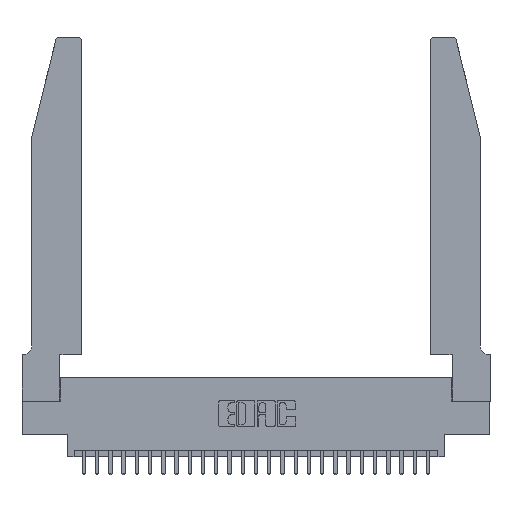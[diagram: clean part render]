
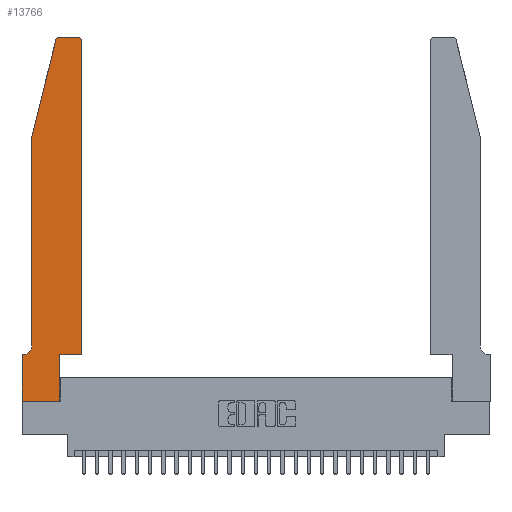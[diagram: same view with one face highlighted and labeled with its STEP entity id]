
A CAD part, top view. The second image highlights one B-rep face of the part: STEP entity #13766.
In plain terms, the highlighted planar face has unit normal (0, 0, 1).
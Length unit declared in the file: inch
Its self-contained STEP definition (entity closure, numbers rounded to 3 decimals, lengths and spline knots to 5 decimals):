
#180 = VECTOR ( 'NONE', #20791, 39.37008 ) ;
#349 = CARTESIAN_POINT ( 'NONE',  ( 0.0055, 0.35, 0.37 ) ) ;
#538 = DIRECTION ( 'NONE',  ( 0., 0., 1. ) ) ;
#613 = DIRECTION ( 'NONE',  ( -0.239, -0.971, 0. ) ) ;
#856 = CARTESIAN_POINT ( 'NONE',  ( 0.2605, 2.75, 0.37 ) ) ;
#1047 = EDGE_CURVE ( 'NONE', #24297, #16888, #28134, .T. ) ;
#1072 = DIRECTION ( 'NONE',  ( 0., 1., 0. ) ) ;
#1784 = CARTESIAN_POINT ( 'NONE',  ( 0., 0., 0.37 ) ) ;
#1854 = VECTOR ( 'NONE', #25260, 39.37008 ) ;
#2248 = EDGE_CURVE ( 'NONE', #17133, #15764, #22251, .T. ) ;
#2498 = VERTEX_POINT ( 'NONE', #10801 ) ;
#3468 = CIRCLE ( 'NONE', #11384, 0.03 ) ;
#3705 = DIRECTION ( 'NONE',  ( 1., 0., 0. ) ) ;
#4107 = AXIS2_PLACEMENT_3D ( 'NONE', #14179, #20721, #8037 ) ;
#4218 = CARTESIAN_POINT ( 'NONE',  ( 0.0755, 2., 0.37 ) ) ;
#4398 = EDGE_CURVE ( 'NONE', #16888, #2498, #3468, .T. ) ;
#4449 = CARTESIAN_POINT ( 'NONE',  ( 0.0755, 0.35, 0.37 ) ) ;
#4820 = VECTOR ( 'NONE', #8556, 39.37008 ) ;
#5289 = ORIENTED_EDGE ( 'NONE', *, *, #16369, .T. ) ;
#6304 = LINE ( 'NONE', #22009, #22930 ) ;
#6867 = CARTESIAN_POINT ( 'NONE',  ( 0., 0.35, 0.37 ) ) ;
#7314 = VECTOR ( 'NONE', #1072, 39.37008 ) ;
#7730 = CARTESIAN_POINT ( 'NONE',  ( 0.0755, 2., 0.37 ) ) ;
#8037 = DIRECTION ( 'NONE',  ( -1., 0., 0. ) ) ;
#8048 = VECTOR ( 'NONE', #26837, 39.37008 ) ;
#8246 = CARTESIAN_POINT ( 'NONE',  ( 0., 0.35, 0.37 ) ) ;
#8325 = VERTEX_POINT ( 'NONE', #9716 ) ;
#8399 = LINE ( 'NONE', #27541, #14498 ) ;
#8482 = DIRECTION ( 'NONE',  ( 1., 0., 0. ) ) ;
#8556 = DIRECTION ( 'NONE',  ( 1., 0., 0. ) ) ;
#8605 = ORIENTED_EDGE ( 'NONE', *, *, #16650, .T. ) ;
#9026 = CARTESIAN_POINT ( 'NONE',  ( 0.2865, 0.35, 0.37 ) ) ;
#9716 = CARTESIAN_POINT ( 'NONE',  ( 0.0755, 2., 0.37 ) ) ;
#9891 = CARTESIAN_POINT ( 'NONE',  ( 0.2865, 0., 0.37 ) ) ;
#10293 = ORIENTED_EDGE ( 'NONE', *, *, #2248, .T. ) ;
#10742 = LINE ( 'NONE', #20646, #8048 ) ;
#10801 = CARTESIAN_POINT ( 'NONE',  ( 0.25487, 2.72718, 0.37 ) ) ;
#10845 = ORIENTED_EDGE ( 'NONE', *, *, #22324, .T. ) ;
#10915 = ORIENTED_EDGE ( 'NONE', *, *, #21573, .T. ) ;
#11346 = CARTESIAN_POINT ( 'NONE',  ( 0.4205, 2.72, 0.37 ) ) ;
#11384 = AXIS2_PLACEMENT_3D ( 'NONE', #19476, #27945, #8482 ) ;
#11965 = EDGE_CURVE ( 'NONE', #21100, #16824, #18745, .T. ) ;
#12116 = ORIENTED_EDGE ( 'NONE', *, *, #24431, .T. ) ;
#12327 = VERTEX_POINT ( 'NONE', #9891 ) ;
#12569 = CARTESIAN_POINT ( 'NONE',  ( 0.284, 2.75, 0.37 ) ) ;
#13395 = LINE ( 'NONE', #4449, #1854 ) ;
#13766 = ADVANCED_FACE ( 'NONE', ( #23053 ), #27431, .T. ) ;
#14179 = CARTESIAN_POINT ( 'NONE',  ( 0.0055, 0.42, 0.37 ) ) ;
#14498 = VECTOR ( 'NONE', #27365, 39.37008 ) ;
#15276 = EDGE_CURVE ( 'NONE', #12327, #16425, #8399, .T. ) ;
#15707 = CIRCLE ( 'NONE', #15959, 0.03 ) ;
#15764 = VERTEX_POINT ( 'NONE', #24985 ) ;
#15841 = VECTOR ( 'NONE', #613, 39.37008 ) ;
#15959 = AXIS2_PLACEMENT_3D ( 'NONE', #11346, #538, #17813 ) ;
#16176 = VERTEX_POINT ( 'NONE', #6867 ) ;
#16369 = EDGE_CURVE ( 'NONE', #16176, #26821, #6304, .T. ) ;
#16425 = VERTEX_POINT ( 'NONE', #9026 ) ;
#16543 = ORIENTED_EDGE ( 'NONE', *, *, #1047, .T. ) ;
#16650 = EDGE_CURVE ( 'NONE', #16824, #16176, #13395, .T. ) ;
#16824 = VERTEX_POINT ( 'NONE', #349 ) ;
#16888 = VERTEX_POINT ( 'NONE', #12569 ) ;
#17133 = VERTEX_POINT ( 'NONE', #24877 ) ;
#17414 = ORIENTED_EDGE ( 'NONE', *, *, #11965, .T. ) ;
#17813 = DIRECTION ( 'NONE',  ( 1., 0., 0. ) ) ;
#18031 = LINE ( 'NONE', #23453, #4820 ) ;
#18745 = CIRCLE ( 'NONE', #4107, 0.07 ) ;
#19476 = CARTESIAN_POINT ( 'NONE',  ( 0.284, 2.72, 0.37 ) ) ;
#19830 = DIRECTION ( 'NONE',  ( 0., -1., 0. ) ) ;
#20646 = CARTESIAN_POINT ( 'NONE',  ( 0.4505, 0.35, 0.37 ) ) ;
#20721 = DIRECTION ( 'NONE',  ( 0., 0., -1. ) ) ;
#20791 = DIRECTION ( 'NONE',  ( 0., -1., 0. ) ) ;
#20929 = LINE ( 'NONE', #4218, #15841 ) ;
#20981 = VECTOR ( 'NONE', #26876, 39.37008 ) ;
#21100 = VERTEX_POINT ( 'NONE', #27762 ) ;
#21184 = CARTESIAN_POINT ( 'NONE',  ( 0.4205, 2.75, 0.37 ) ) ;
#21460 = EDGE_CURVE ( 'NONE', #2498, #8325, #20929, .T. ) ;
#21573 = EDGE_CURVE ( 'NONE', #16425, #17133, #10742, .T. ) ;
#22009 = CARTESIAN_POINT ( 'NONE',  ( 0., 0., 0.37 ) ) ;
#22251 = LINE ( 'NONE', #27095, #7314 ) ;
#22324 = EDGE_CURVE ( 'NONE', #8325, #21100, #28021, .T. ) ;
#22930 = VECTOR ( 'NONE', #19830, 39.37008 ) ;
#23053 = FACE_OUTER_BOUND ( 'NONE', #25169, .T. ) ;
#23130 = DIRECTION ( 'NONE',  ( 0., 0., 1. ) ) ;
#23453 = CARTESIAN_POINT ( 'NONE',  ( 0., 0., 0.37 ) ) ;
#24297 = VERTEX_POINT ( 'NONE', #21184 ) ;
#24431 = EDGE_CURVE ( 'NONE', #26821, #12327, #18031, .T. ) ;
#24877 = CARTESIAN_POINT ( 'NONE',  ( 0.4505, 0.35, 0.37 ) ) ;
#24985 = CARTESIAN_POINT ( 'NONE',  ( 0.4505, 2.72, 0.37 ) ) ;
#25169 = EDGE_LOOP ( 'NONE', ( #16543, #25795, #25271, #10845, #17414, #8605, #5289, #12116, #27319, #10915, #10293, #25614 ) ) ;
#25260 = DIRECTION ( 'NONE',  ( -1., 0., 0. ) ) ;
#25271 = ORIENTED_EDGE ( 'NONE', *, *, #21460, .T. ) ;
#25503 = EDGE_CURVE ( 'NONE', #15764, #24297, #15707, .T. ) ;
#25614 = ORIENTED_EDGE ( 'NONE', *, *, #25503, .T. ) ;
#25795 = ORIENTED_EDGE ( 'NONE', *, *, #4398, .T. ) ;
#26284 = AXIS2_PLACEMENT_3D ( 'NONE', #8246, #23130, #3705 ) ;
#26821 = VERTEX_POINT ( 'NONE', #1784 ) ;
#26837 = DIRECTION ( 'NONE',  ( 1., 0., 0. ) ) ;
#26876 = DIRECTION ( 'NONE',  ( -1., 0., 0. ) ) ;
#27095 = CARTESIAN_POINT ( 'NONE',  ( 0.4505, 0.35, 0.37 ) ) ;
#27319 = ORIENTED_EDGE ( 'NONE', *, *, #15276, .T. ) ;
#27365 = DIRECTION ( 'NONE',  ( 0., 1., 0. ) ) ;
#27431 = PLANE ( 'NONE',  #26284 ) ;
#27541 = CARTESIAN_POINT ( 'NONE',  ( 0.2865, 0.35, 0.37 ) ) ;
#27762 = CARTESIAN_POINT ( 'NONE',  ( 0.0755, 0.42, 0.37 ) ) ;
#27945 = DIRECTION ( 'NONE',  ( 0., 0., 1. ) ) ;
#28021 = LINE ( 'NONE', #7730, #180 ) ;
#28134 = LINE ( 'NONE', #856, #20981 ) ;
